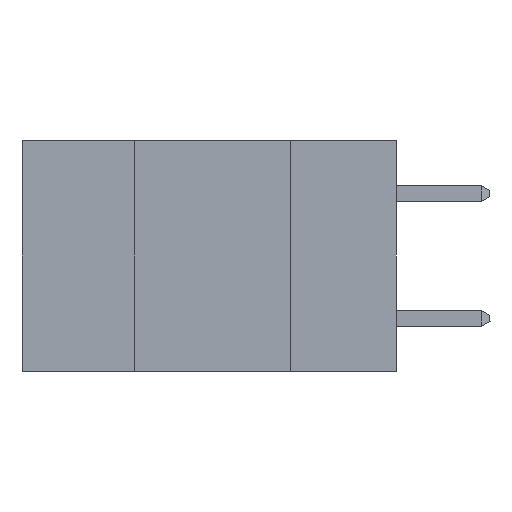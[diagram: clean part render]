
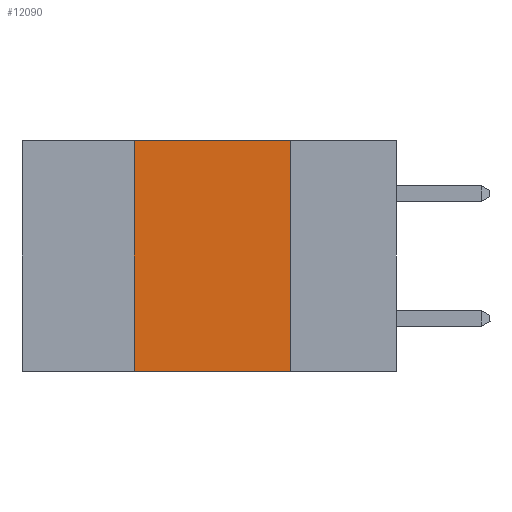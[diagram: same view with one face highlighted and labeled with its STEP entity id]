
A CAD part, left-side view. The second image highlights one B-rep face of the part: STEP entity #12090.
In plain terms, the highlighted planar face has unit normal (-1, 0, 0).
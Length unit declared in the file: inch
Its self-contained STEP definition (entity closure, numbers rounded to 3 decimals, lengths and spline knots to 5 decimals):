
#858 = CARTESIAN_POINT ( 'NONE',  ( 0., 0.6, 0. ) ) ;
#1849 = CARTESIAN_POINT ( 'NONE',  ( 0., 0.17, 0. ) ) ;
#1860 = CARTESIAN_POINT ( 'NONE',  ( 0., 0.17, -0.37 ) ) ;
#2133 = ORIENTED_EDGE ( 'NONE', *, *, #16018, .F. ) ;
#2304 = DIRECTION ( 'NONE',  ( 0., -1., 0. ) ) ;
#2638 = VERTEX_POINT ( 'NONE', #3505 ) ;
#2847 = PLANE ( 'NONE',  #15735 ) ;
#3477 = ORIENTED_EDGE ( 'NONE', *, *, #22346, .F. ) ;
#3505 = CARTESIAN_POINT ( 'NONE',  ( 0., 0.17, -0.37 ) ) ;
#3525 = EDGE_CURVE ( 'NONE', #3964, #2638, #7928, .T. ) ;
#3822 = DIRECTION ( 'NONE',  ( 0., 0., -1. ) ) ;
#3845 = LINE ( 'NONE', #23223, #22297 ) ;
#3964 = VERTEX_POINT ( 'NONE', #22605 ) ;
#4230 = CARTESIAN_POINT ( 'NONE',  ( 0., 0.6, -0.37 ) ) ;
#4729 = LINE ( 'NONE', #24260, #9255 ) ;
#4804 = DIRECTION ( 'NONE',  ( 0., 0., -1. ) ) ;
#5271 = VECTOR ( 'NONE', #3822, 39.37008 ) ;
#5317 = DIRECTION ( 'NONE',  ( 0., 0., 1. ) ) ;
#5539 = VERTEX_POINT ( 'NONE', #23315 ) ;
#5711 = EDGE_LOOP ( 'NONE', ( #3477, #15711, #2133, #11769 ) ) ;
#7928 = LINE ( 'NONE', #4230, #18532 ) ;
#8544 = FACE_OUTER_BOUND ( 'NONE', #5711, .T. ) ;
#9255 = VECTOR ( 'NONE', #5317, 39.37008 ) ;
#9291 = VERTEX_POINT ( 'NONE', #1849 ) ;
#11769 = ORIENTED_EDGE ( 'NONE', *, *, #3525, .T. ) ;
#12090 = ADVANCED_FACE ( 'NONE', ( #8544 ), #2847, .F. ) ;
#15393 = LINE ( 'NONE', #1860, #5271 ) ;
#15711 = ORIENTED_EDGE ( 'NONE', *, *, #19772, .F. ) ;
#15735 = AXIS2_PLACEMENT_3D ( 'NONE', #858, #16199, #4804 ) ;
#16018 = EDGE_CURVE ( 'NONE', #3964, #5539, #4729, .T. ) ;
#16199 = DIRECTION ( 'NONE',  ( 1., 0., 0. ) ) ;
#18532 = VECTOR ( 'NONE', #23210, 39.37008 ) ;
#19772 = EDGE_CURVE ( 'NONE', #5539, #9291, #3845, .T. ) ;
#22297 = VECTOR ( 'NONE', #2304, 39.37008 ) ;
#22346 = EDGE_CURVE ( 'NONE', #9291, #2638, #15393, .T. ) ;
#22605 = CARTESIAN_POINT ( 'NONE',  ( 0., 0.42, -0.37 ) ) ;
#23210 = DIRECTION ( 'NONE',  ( 0., -1., 0. ) ) ;
#23223 = CARTESIAN_POINT ( 'NONE',  ( 0., 0.6, 0. ) ) ;
#23315 = CARTESIAN_POINT ( 'NONE',  ( 0., 0.42, 0. ) ) ;
#24260 = CARTESIAN_POINT ( 'NONE',  ( 0., 0.42, -0.37 ) ) ;
